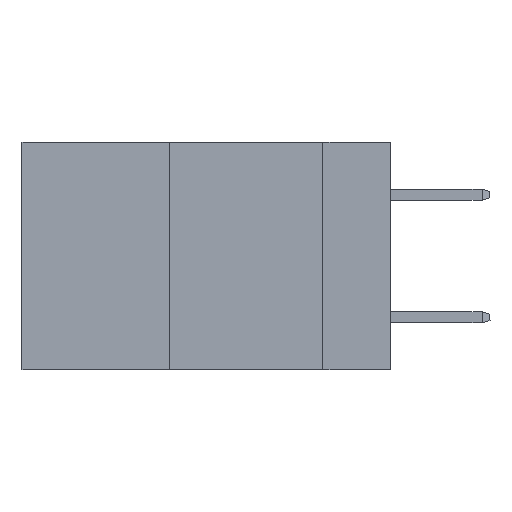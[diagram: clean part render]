
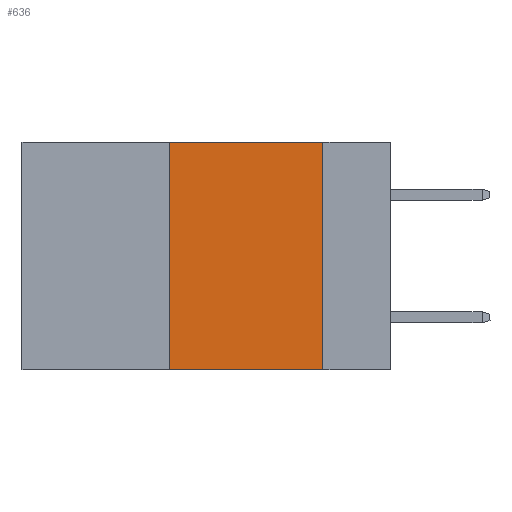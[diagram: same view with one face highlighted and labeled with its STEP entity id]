
A CAD part, left-side view. The second image highlights one B-rep face of the part: STEP entity #636.
In plain terms, the highlighted planar face has unit normal (-1, 0, 0).
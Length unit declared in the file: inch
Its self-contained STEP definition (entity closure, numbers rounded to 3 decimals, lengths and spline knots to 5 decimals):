
#66 = CARTESIAN_POINT ( 'NONE',  ( 0., 0.6, 0. ) ) ;
#82 = DIRECTION ( 'NONE',  ( 0., -1., 0. ) ) ;
#345 = EDGE_CURVE ( 'NONE', #10654, #1534, #1935, .T. ) ;
#347 = VERTEX_POINT ( 'NONE', #1986 ) ;
#636 = ADVANCED_FACE ( 'NONE', ( #7884 ), #2516, .F. ) ;
#714 = AXIS2_PLACEMENT_3D ( 'NONE', #11562, #4177, #6830 ) ;
#1101 = DIRECTION ( 'NONE',  ( 0., -1., 0. ) ) ;
#1414 = VECTOR ( 'NONE', #8137, 39.37008 ) ;
#1534 = VERTEX_POINT ( 'NONE', #4039 ) ;
#1935 = LINE ( 'NONE', #5720, #6517 ) ;
#1972 = ORIENTED_EDGE ( 'NONE', *, *, #345, .F. ) ;
#1986 = CARTESIAN_POINT ( 'NONE',  ( 0., 0.11, -0.37 ) ) ;
#2082 = DIRECTION ( 'NONE',  ( 0., 0., 1. ) ) ;
#2516 = PLANE ( 'NONE',  #714 ) ;
#2598 = VECTOR ( 'NONE', #1101, 39.37008 ) ;
#2738 = CARTESIAN_POINT ( 'NONE',  ( 0., 0.36, -0.37 ) ) ;
#4039 = CARTESIAN_POINT ( 'NONE',  ( 0., 0.36, 0. ) ) ;
#4177 = DIRECTION ( 'NONE',  ( 1., 0., 0. ) ) ;
#4437 = ORIENTED_EDGE ( 'NONE', *, *, #6006, .T. ) ;
#4482 = ORIENTED_EDGE ( 'NONE', *, *, #6644, .F. ) ;
#5105 = CARTESIAN_POINT ( 'NONE',  ( 0., 0.11, 0. ) ) ;
#5720 = CARTESIAN_POINT ( 'NONE',  ( 0., 0.36, 0. ) ) ;
#6006 = EDGE_CURVE ( 'NONE', #10654, #347, #8583, .T. ) ;
#6214 = VECTOR ( 'NONE', #82, 39.37008 ) ;
#6420 = EDGE_LOOP ( 'NONE', ( #9429, #4482, #1972, #4437 ) ) ;
#6517 = VECTOR ( 'NONE', #2082, 39.37008 ) ;
#6644 = EDGE_CURVE ( 'NONE', #1534, #10302, #9426, .T. ) ;
#6830 = DIRECTION ( 'NONE',  ( 0., 0., -1. ) ) ;
#7884 = FACE_OUTER_BOUND ( 'NONE', #6420, .T. ) ;
#8137 = DIRECTION ( 'NONE',  ( 0., 0., -1. ) ) ;
#8583 = LINE ( 'NONE', #10962, #6214 ) ;
#9426 = LINE ( 'NONE', #66, #2598 ) ;
#9429 = ORIENTED_EDGE ( 'NONE', *, *, #9797, .F. ) ;
#9797 = EDGE_CURVE ( 'NONE', #10302, #347, #11204, .T. ) ;
#10302 = VERTEX_POINT ( 'NONE', #5105 ) ;
#10654 = VERTEX_POINT ( 'NONE', #2738 ) ;
#10962 = CARTESIAN_POINT ( 'NONE',  ( 0., 0.6, -0.37 ) ) ;
#11204 = LINE ( 'NONE', #11524, #1414 ) ;
#11524 = CARTESIAN_POINT ( 'NONE',  ( 0., 0.11, 0. ) ) ;
#11562 = CARTESIAN_POINT ( 'NONE',  ( 0., 0.6, 0. ) ) ;
